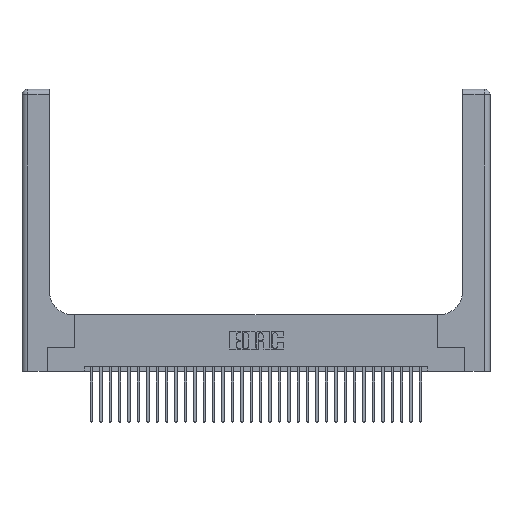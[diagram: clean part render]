
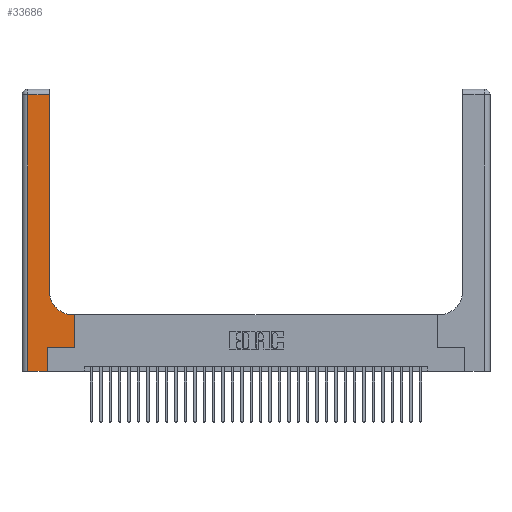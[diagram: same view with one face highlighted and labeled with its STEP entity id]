
A CAD part, top view. The second image highlights one B-rep face of the part: STEP entity #33686.
In plain terms, the highlighted planar face has unit normal (0, 0, 1).
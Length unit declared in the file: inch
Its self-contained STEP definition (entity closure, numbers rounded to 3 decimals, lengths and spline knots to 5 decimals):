
#68 = LINE ( 'NONE', #2192, #31162 ) ;
#1126 = VERTEX_POINT ( 'NONE', #32623 ) ;
#1199 = EDGE_CURVE ( 'NONE', #29812, #11051, #33886, .T. ) ;
#1266 = VECTOR ( 'NONE', #15105, 39.37008 ) ;
#1567 = DIRECTION ( 'NONE',  ( 1., 0., 0. ) ) ;
#1711 = CARTESIAN_POINT ( 'NONE',  ( 0.5585, 0.25, 0.37 ) ) ;
#1870 = LINE ( 'NONE', #12749, #22963 ) ;
#2002 = VERTEX_POINT ( 'NONE', #26866 ) ;
#2192 = CARTESIAN_POINT ( 'NONE',  ( 0., 2.94, 0.37 ) ) ;
#2216 = EDGE_CURVE ( 'NONE', #11051, #19570, #30035, .T. ) ;
#2791 = EDGE_CURVE ( 'NONE', #22650, #4802, #32481, .T. ) ;
#2843 = EDGE_CURVE ( 'NONE', #4802, #2002, #1870, .T. ) ;
#4607 = AXIS2_PLACEMENT_3D ( 'NONE', #34219, #10434, #23454 ) ;
#4802 = VERTEX_POINT ( 'NONE', #23495 ) ;
#6176 = CARTESIAN_POINT ( 'NONE',  ( 0.5585, 0.25, 0.37 ) ) ;
#6464 = ORIENTED_EDGE ( 'NONE', *, *, #7253, .T. ) ;
#6738 = VERTEX_POINT ( 'NONE', #32527 ) ;
#6831 = EDGE_CURVE ( 'NONE', #12911, #6738, #22350, .T. ) ;
#7198 = PLANE ( 'NONE',  #33639 ) ;
#7253 = EDGE_CURVE ( 'NONE', #19570, #1126, #17011, .T. ) ;
#7915 = DIRECTION ( 'NONE',  ( -1., 0., 0. ) ) ;
#8364 = LINE ( 'NONE', #22899, #1266 ) ;
#8566 = ORIENTED_EDGE ( 'NONE', *, *, #6831, .T. ) ;
#9302 = VECTOR ( 'NONE', #24370, 39.37008 ) ;
#9880 = DIRECTION ( 'NONE',  ( 0., 0., -1. ) ) ;
#9997 = ORIENTED_EDGE ( 'NONE', *, *, #2843, .T. ) ;
#10268 = VECTOR ( 'NONE', #1567, 39.37008 ) ;
#10434 = DIRECTION ( 'NONE',  ( 0., 0., -1. ) ) ;
#11051 = VERTEX_POINT ( 'NONE', #12476 ) ;
#11077 = ORIENTED_EDGE ( 'NONE', *, *, #1199, .T. ) ;
#12374 = FACE_OUTER_BOUND ( 'NONE', #31899, .T. ) ;
#12476 = CARTESIAN_POINT ( 'NONE',  ( 0.269, 0.25, 0.37 ) ) ;
#12749 = CARTESIAN_POINT ( 'NONE',  ( 0.2915, 3., 0.37 ) ) ;
#12861 = DIRECTION ( 'NONE',  ( 0., 1., 0. ) ) ;
#12911 = VERTEX_POINT ( 'NONE', #16726 ) ;
#14703 = LINE ( 'NONE', #27367, #9302 ) ;
#14816 = CARTESIAN_POINT ( 'NONE',  ( 0.269, 0.25, 0.37 ) ) ;
#15105 = DIRECTION ( 'NONE',  ( -1., 0., 0. ) ) ;
#16388 = ORIENTED_EDGE ( 'NONE', *, *, #16511, .T. ) ;
#16511 = EDGE_CURVE ( 'NONE', #6738, #29812, #14703, .T. ) ;
#16726 = CARTESIAN_POINT ( 'NONE',  ( 0.06, 2.94, 0.37 ) ) ;
#17011 = LINE ( 'NONE', #1711, #32277 ) ;
#17603 = CARTESIAN_POINT ( 'NONE',  ( 0., 3., 0.37 ) ) ;
#17804 = CARTESIAN_POINT ( 'NONE',  ( 0.06, 3., 0.37 ) ) ;
#18972 = ORIENTED_EDGE ( 'NONE', *, *, #30880, .T. ) ;
#19063 = EDGE_CURVE ( 'NONE', #2002, #12911, #68, .T. ) ;
#19379 = DIRECTION ( 'NONE',  ( 0., 1., 0. ) ) ;
#19570 = VERTEX_POINT ( 'NONE', #6176 ) ;
#20562 = ORIENTED_EDGE ( 'NONE', *, *, #2216, .T. ) ;
#22350 = LINE ( 'NONE', #17804, #33574 ) ;
#22650 = VERTEX_POINT ( 'NONE', #24625 ) ;
#22899 = CARTESIAN_POINT ( 'NONE',  ( 0.2915, 0.6, 0.37 ) ) ;
#22963 = VECTOR ( 'NONE', #12861, 39.37008 ) ;
#23454 = DIRECTION ( 'NONE',  ( 1., 0., 0. ) ) ;
#23495 = CARTESIAN_POINT ( 'NONE',  ( 0.2915, 0.85, 0.37 ) ) ;
#23658 = CARTESIAN_POINT ( 'NONE',  ( 0.269, 0., 0.37 ) ) ;
#24370 = DIRECTION ( 'NONE',  ( 1., 0., 0. ) ) ;
#24625 = CARTESIAN_POINT ( 'NONE',  ( 0.5415, 0.6, 0.37 ) ) ;
#25046 = DIRECTION ( 'NONE',  ( 0., 1., 0. ) ) ;
#26866 = CARTESIAN_POINT ( 'NONE',  ( 0.2915, 2.94, 0.37 ) ) ;
#26882 = CARTESIAN_POINT ( 'NONE',  ( 0.269, 0., 0.37 ) ) ;
#27367 = CARTESIAN_POINT ( 'NONE',  ( 0., 0., 0.37 ) ) ;
#28085 = VECTOR ( 'NONE', #19379, 39.37008 ) ;
#28309 = DIRECTION ( 'NONE',  ( -1., 0., 0. ) ) ;
#29812 = VERTEX_POINT ( 'NONE', #23658 ) ;
#30035 = LINE ( 'NONE', #14816, #10268 ) ;
#30880 = EDGE_CURVE ( 'NONE', #1126, #22650, #8364, .T. ) ;
#31162 = VECTOR ( 'NONE', #7915, 39.37008 ) ;
#31204 = ORIENTED_EDGE ( 'NONE', *, *, #19063, .T. ) ;
#31643 = ORIENTED_EDGE ( 'NONE', *, *, #2791, .T. ) ;
#31899 = EDGE_LOOP ( 'NONE', ( #9997, #31204, #8566, #16388, #11077, #20562, #6464, #18972, #31643 ) ) ;
#32277 = VECTOR ( 'NONE', #25046, 39.37008 ) ;
#32481 = CIRCLE ( 'NONE', #4607, 0.25 ) ;
#32527 = CARTESIAN_POINT ( 'NONE',  ( 0.06, 0., 0.37 ) ) ;
#32623 = CARTESIAN_POINT ( 'NONE',  ( 0.5585, 0.6, 0.37 ) ) ;
#33574 = VECTOR ( 'NONE', #33710, 39.37008 ) ;
#33639 = AXIS2_PLACEMENT_3D ( 'NONE', #17603, #9880, #28309 ) ;
#33686 = ADVANCED_FACE ( 'NONE', ( #12374 ), #7198, .F. ) ;
#33710 = DIRECTION ( 'NONE',  ( 0., -1., 0. ) ) ;
#33886 = LINE ( 'NONE', #26882, #28085 ) ;
#34219 = CARTESIAN_POINT ( 'NONE',  ( 0.5415, 0.85, 0.37 ) ) ;
